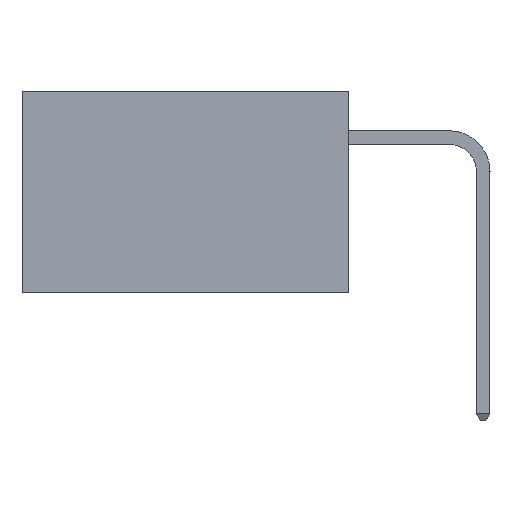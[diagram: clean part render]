
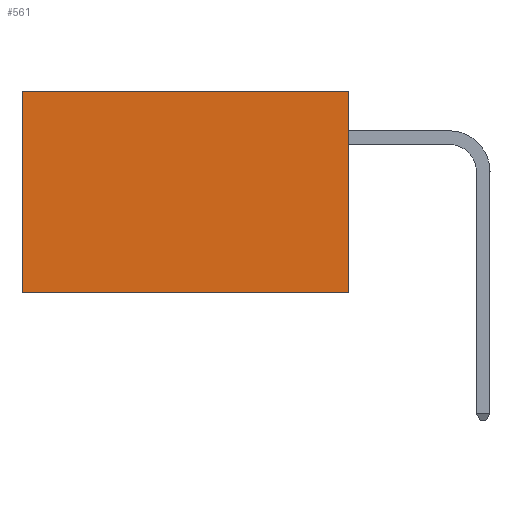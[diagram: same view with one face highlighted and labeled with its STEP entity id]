
A CAD part, left-side view. The second image highlights one B-rep face of the part: STEP entity #561.
In plain terms, the highlighted planar face has unit normal (-1, 0, 0).
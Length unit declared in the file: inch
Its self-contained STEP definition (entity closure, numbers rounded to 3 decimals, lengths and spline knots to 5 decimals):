
#255 = ORIENTED_EDGE ( 'NONE', *, *, #13009, .T. ) ;
#561 = ADVANCED_FACE ( 'NONE', ( #10608 ), #16126, .F. ) ;
#997 = VERTEX_POINT ( 'NONE', #6235 ) ;
#1621 = CARTESIAN_POINT ( 'NONE',  ( 0.2875, 0., 0. ) ) ;
#2204 = ORIENTED_EDGE ( 'NONE', *, *, #16914, .F. ) ;
#2812 = CARTESIAN_POINT ( 'NONE',  ( 0.2875, 0.6, 0. ) ) ;
#2921 = ORIENTED_EDGE ( 'NONE', *, *, #12438, .T. ) ;
#3447 = ORIENTED_EDGE ( 'NONE', *, *, #7263, .F. ) ;
#4432 = VERTEX_POINT ( 'NONE', #15016 ) ;
#4648 = CARTESIAN_POINT ( 'NONE',  ( 0.2875, 0., 0. ) ) ;
#5229 = CARTESIAN_POINT ( 'NONE',  ( 0.2875, 0., -0.37 ) ) ;
#6235 = CARTESIAN_POINT ( 'NONE',  ( 0.2875, 0.6, -0.37 ) ) ;
#6308 = DIRECTION ( 'NONE',  ( 0., 1., 0. ) ) ;
#6987 = LINE ( 'NONE', #5229, #19617 ) ;
#7263 = EDGE_CURVE ( 'NONE', #15969, #7570, #16192, .T. ) ;
#7570 = VERTEX_POINT ( 'NONE', #20135 ) ;
#8108 = AXIS2_PLACEMENT_3D ( 'NONE', #1621, #19352, #14812 ) ;
#10608 = FACE_OUTER_BOUND ( 'NONE', #12519, .T. ) ;
#12001 = VECTOR ( 'NONE', #16249, 39.37008 ) ;
#12248 = VECTOR ( 'NONE', #12551, 39.37008 ) ;
#12438 = EDGE_CURVE ( 'NONE', #15969, #4432, #19896, .T. ) ;
#12519 = EDGE_LOOP ( 'NONE', ( #255, #2204, #3447, #2921 ) ) ;
#12551 = DIRECTION ( 'NONE',  ( 0., 0., -1. ) ) ;
#13009 = EDGE_CURVE ( 'NONE', #4432, #997, #16934, .T. ) ;
#13306 = DIRECTION ( 'NONE',  ( 0., 1., 0. ) ) ;
#14637 = CARTESIAN_POINT ( 'NONE',  ( 0.2875, 0., 0. ) ) ;
#14812 = DIRECTION ( 'NONE',  ( 0., 0., -1. ) ) ;
#15016 = CARTESIAN_POINT ( 'NONE',  ( 0.2875, 0.6, 0. ) ) ;
#15969 = VERTEX_POINT ( 'NONE', #16324 ) ;
#16126 = PLANE ( 'NONE',  #8108 ) ;
#16192 = LINE ( 'NONE', #14637, #12001 ) ;
#16249 = DIRECTION ( 'NONE',  ( 0., 0., -1. ) ) ;
#16324 = CARTESIAN_POINT ( 'NONE',  ( 0.2875, 0., 0. ) ) ;
#16914 = EDGE_CURVE ( 'NONE', #7570, #997, #6987, .T. ) ;
#16934 = LINE ( 'NONE', #2812, #12248 ) ;
#19352 = DIRECTION ( 'NONE',  ( 1., 0., 0. ) ) ;
#19617 = VECTOR ( 'NONE', #13306, 39.37008 ) ;
#19896 = LINE ( 'NONE', #4648, #20383 ) ;
#20135 = CARTESIAN_POINT ( 'NONE',  ( 0.2875, 0., -0.37 ) ) ;
#20383 = VECTOR ( 'NONE', #6308, 39.37008 ) ;
